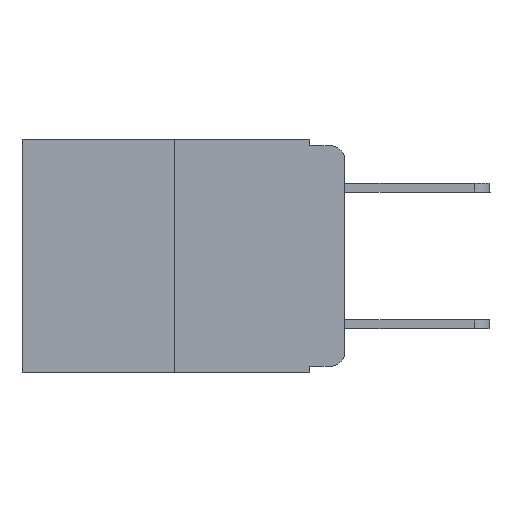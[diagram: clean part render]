
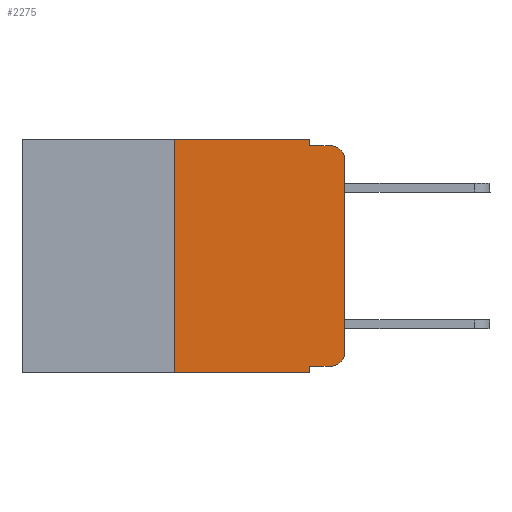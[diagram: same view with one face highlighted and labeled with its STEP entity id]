
A CAD part, left-side view. The second image highlights one B-rep face of the part: STEP entity #2275.
In plain terms, the highlighted planar face has unit normal (-1, 0, 0).
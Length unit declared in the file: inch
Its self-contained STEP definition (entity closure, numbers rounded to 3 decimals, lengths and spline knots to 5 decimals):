
#175 = CARTESIAN_POINT ( 'NONE',  ( 0., 0., -0.313 ) ) ;
#224 = DIRECTION ( 'NONE',  ( 0., 0., 1. ) ) ;
#630 = PLANE ( 'NONE',  #7409 ) ;
#812 = AXIS2_PLACEMENT_3D ( 'NONE', #2755, #3411, #7139 ) ;
#1079 = LINE ( 'NONE', #2976, #1802 ) ;
#1200 = VERTEX_POINT ( 'NONE', #7277 ) ;
#1433 = LINE ( 'NONE', #7550, #6751 ) ;
#1802 = VECTOR ( 'NONE', #3745, 39.37008 ) ;
#1962 = DIRECTION ( 'NONE',  ( 0., 0., -1. ) ) ;
#2109 = VERTEX_POINT ( 'NONE', #9494 ) ;
#2128 = AXIS2_PLACEMENT_3D ( 'NONE', #7150, #4223, #1962 ) ;
#2156 = DIRECTION ( 'NONE',  ( 0., 0., -1. ) ) ;
#2217 = DIRECTION ( 'NONE',  ( 0., -1., 0. ) ) ;
#2275 = ADVANCED_FACE ( 'NONE', ( #6850 ), #630, .F. ) ;
#2590 = CARTESIAN_POINT ( 'NONE',  ( 0., 0.051, -0.01 ) ) ;
#2693 = EDGE_CURVE ( 'NONE', #9213, #8272, #5256, .T. ) ;
#2747 = EDGE_CURVE ( 'NONE', #3284, #2109, #7003, .T. ) ;
#2755 = CARTESIAN_POINT ( 'NONE',  ( 0., 0.02, -0.313 ) ) ;
#2767 = LINE ( 'NONE', #9251, #8883 ) ;
#2931 = VERTEX_POINT ( 'NONE', #8789 ) ;
#2942 = EDGE_CURVE ( 'NONE', #3284, #5963, #6334, .T. ) ;
#2976 = CARTESIAN_POINT ( 'NONE',  ( 0., 0.473, 0. ) ) ;
#3145 = VERTEX_POINT ( 'NONE', #2590 ) ;
#3246 = EDGE_CURVE ( 'NONE', #8690, #1200, #3251, .T. ) ;
#3251 = CIRCLE ( 'NONE', #2128, 0.02 ) ;
#3284 = VERTEX_POINT ( 'NONE', #5776 ) ;
#3411 = DIRECTION ( 'NONE',  ( -1., 0., 0. ) ) ;
#3552 = DIRECTION ( 'NONE',  ( 0., 0., 1. ) ) ;
#3604 = DIRECTION ( 'NONE',  ( 0., 0., -1. ) ) ;
#3641 = CARTESIAN_POINT ( 'NONE',  ( 0., 0.473, 0. ) ) ;
#3692 = DIRECTION ( 'NONE',  ( 0., -1., 0. ) ) ;
#3745 = DIRECTION ( 'NONE',  ( 0., -1., 0. ) ) ;
#3805 = ORIENTED_EDGE ( 'NONE', *, *, #2747, .T. ) ;
#3835 = EDGE_CURVE ( 'NONE', #5517, #2109, #4189, .T. ) ;
#3972 = CARTESIAN_POINT ( 'NONE',  ( 0., 0.051, 0. ) ) ;
#4189 = LINE ( 'NONE', #8859, #6553 ) ;
#4223 = DIRECTION ( 'NONE',  ( -1., 0., 0. ) ) ;
#4344 = CARTESIAN_POINT ( 'NONE',  ( 0., 0.25, 0. ) ) ;
#4386 = ORIENTED_EDGE ( 'NONE', *, *, #3835, .F. ) ;
#5256 = CIRCLE ( 'NONE', #812, 0.02 ) ;
#5517 = VERTEX_POINT ( 'NONE', #7972 ) ;
#5705 = EDGE_CURVE ( 'NONE', #3145, #1200, #1433, .T. ) ;
#5723 = VECTOR ( 'NONE', #9489, 39.37008 ) ;
#5738 = CARTESIAN_POINT ( 'NONE',  ( 0., 0.473, -0.343 ) ) ;
#5776 = CARTESIAN_POINT ( 'NONE',  ( 0., 0.25, -0.343 ) ) ;
#5868 = CARTESIAN_POINT ( 'NONE',  ( 0., 0.02, -0.333 ) ) ;
#5963 = VERTEX_POINT ( 'NONE', #7076 ) ;
#5977 = ORIENTED_EDGE ( 'NONE', *, *, #6618, .T. ) ;
#6035 = ORIENTED_EDGE ( 'NONE', *, *, #2693, .T. ) ;
#6140 = DIRECTION ( 'NONE',  ( 0., 0., -1. ) ) ;
#6334 = LINE ( 'NONE', #4344, #9611 ) ;
#6418 = LINE ( 'NONE', #3972, #8159 ) ;
#6553 = VECTOR ( 'NONE', #2156, 39.37008 ) ;
#6568 = DIRECTION ( 'NONE',  ( 1., 0., 0. ) ) ;
#6571 = VECTOR ( 'NONE', #2217, 39.37008 ) ;
#6618 = EDGE_CURVE ( 'NONE', #5517, #9213, #7013, .T. ) ;
#6751 = VECTOR ( 'NONE', #3692, 39.37008 ) ;
#6850 = FACE_OUTER_BOUND ( 'NONE', #7445, .T. ) ;
#7003 = LINE ( 'NONE', #5738, #5723 ) ;
#7013 = LINE ( 'NONE', #8903, #6571 ) ;
#7076 = CARTESIAN_POINT ( 'NONE',  ( 0., 0.25, 0. ) ) ;
#7139 = DIRECTION ( 'NONE',  ( 0., 0., -1. ) ) ;
#7150 = CARTESIAN_POINT ( 'NONE',  ( 0., 0.02, -0.03 ) ) ;
#7153 = EDGE_CURVE ( 'NONE', #8272, #8690, #2767, .T. ) ;
#7277 = CARTESIAN_POINT ( 'NONE',  ( 0., 0.02, -0.01 ) ) ;
#7409 = AXIS2_PLACEMENT_3D ( 'NONE', #3641, #6568, #3604 ) ;
#7436 = ORIENTED_EDGE ( 'NONE', *, *, #5705, .F. ) ;
#7445 = EDGE_LOOP ( 'NONE', ( #9271, #8250, #7436, #9517, #8499, #8117, #3805, #4386, #5977, #6035 ) ) ;
#7484 = EDGE_CURVE ( 'NONE', #5963, #2931, #1079, .T. ) ;
#7550 = CARTESIAN_POINT ( 'NONE',  ( 0., 0.051, -0.01 ) ) ;
#7972 = CARTESIAN_POINT ( 'NONE',  ( 0., 0.051, -0.333 ) ) ;
#8117 = ORIENTED_EDGE ( 'NONE', *, *, #2942, .F. ) ;
#8159 = VECTOR ( 'NONE', #6140, 39.37008 ) ;
#8250 = ORIENTED_EDGE ( 'NONE', *, *, #3246, .T. ) ;
#8263 = EDGE_CURVE ( 'NONE', #2931, #3145, #6418, .T. ) ;
#8272 = VERTEX_POINT ( 'NONE', #175 ) ;
#8499 = ORIENTED_EDGE ( 'NONE', *, *, #7484, .F. ) ;
#8690 = VERTEX_POINT ( 'NONE', #9569 ) ;
#8789 = CARTESIAN_POINT ( 'NONE',  ( 0., 0.051, 0. ) ) ;
#8859 = CARTESIAN_POINT ( 'NONE',  ( 0., 0.051, 0. ) ) ;
#8883 = VECTOR ( 'NONE', #224, 39.37008 ) ;
#8903 = CARTESIAN_POINT ( 'NONE',  ( 0., 0.051, -0.333 ) ) ;
#9213 = VERTEX_POINT ( 'NONE', #5868 ) ;
#9251 = CARTESIAN_POINT ( 'NONE',  ( 0., 0., 0. ) ) ;
#9271 = ORIENTED_EDGE ( 'NONE', *, *, #7153, .T. ) ;
#9489 = DIRECTION ( 'NONE',  ( 0., -1., 0. ) ) ;
#9494 = CARTESIAN_POINT ( 'NONE',  ( 0., 0.051, -0.343 ) ) ;
#9517 = ORIENTED_EDGE ( 'NONE', *, *, #8263, .F. ) ;
#9569 = CARTESIAN_POINT ( 'NONE',  ( 0., 0., -0.03 ) ) ;
#9611 = VECTOR ( 'NONE', #3552, 39.37008 ) ;
